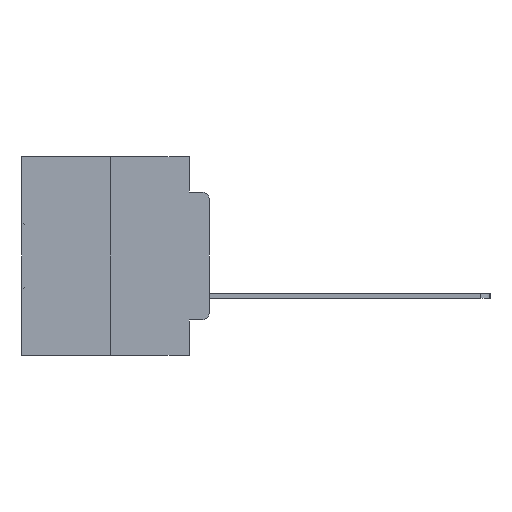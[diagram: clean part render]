
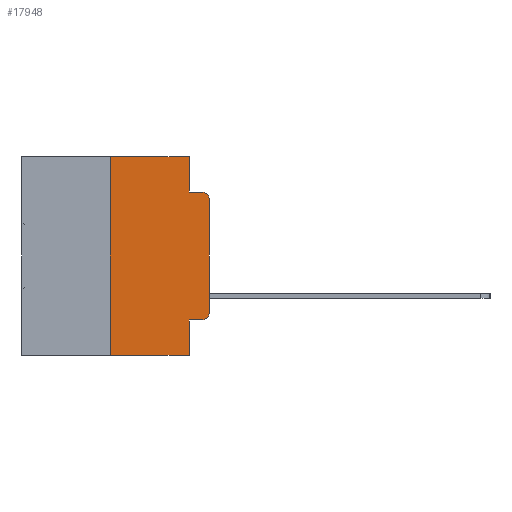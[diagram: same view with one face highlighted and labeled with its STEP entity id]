
A CAD part, left-side view. The second image highlights one B-rep face of the part: STEP entity #17948.
In plain terms, the highlighted planar face has unit normal (-1, 0, 0).
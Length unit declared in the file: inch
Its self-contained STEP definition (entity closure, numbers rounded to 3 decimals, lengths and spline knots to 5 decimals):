
#135 = CARTESIAN_POINT ( 'NONE',  ( 0., 0.473, 0. ) ) ;
#407 = EDGE_CURVE ( 'NONE', #14421, #8506, #14836, .T. ) ;
#2081 = ORIENTED_EDGE ( 'NONE', *, *, #20221, .T. ) ;
#2474 = ORIENTED_EDGE ( 'NONE', *, *, #28296, .F. ) ;
#2685 = DIRECTION ( 'NONE',  ( 0., 0., -1. ) ) ;
#2737 = EDGE_CURVE ( 'NONE', #5109, #17526, #16474, .T. ) ;
#2983 = CARTESIAN_POINT ( 'NONE',  ( 0., 0.473, 0. ) ) ;
#3558 = CARTESIAN_POINT ( 'NONE',  ( 0., 0.25, 0. ) ) ;
#3638 = ORIENTED_EDGE ( 'NONE', *, *, #28166, .T. ) ;
#5041 = EDGE_LOOP ( 'NONE', ( #15099, #5907, #12115, #9415, #2474, #17020, #29614, #31041, #2081, #3638 ) ) ;
#5109 = VERTEX_POINT ( 'NONE', #23077 ) ;
#5199 = DIRECTION ( 'NONE',  ( 0., -1., 0. ) ) ;
#5673 = DIRECTION ( 'NONE',  ( 0., 0., -1. ) ) ;
#5705 = LINE ( 'NONE', #2983, #29736 ) ;
#5858 = CARTESIAN_POINT ( 'NONE',  ( 0., 0.051, 0. ) ) ;
#5907 = ORIENTED_EDGE ( 'NONE', *, *, #24404, .T. ) ;
#5929 = LINE ( 'NONE', #17070, #24414 ) ;
#6015 = EDGE_CURVE ( 'NONE', #12512, #10675, #6375, .T. ) ;
#6375 = LINE ( 'NONE', #15417, #29650 ) ;
#6469 = AXIS2_PLACEMENT_3D ( 'NONE', #23797, #9454, #26210 ) ;
#6505 = VECTOR ( 'NONE', #11482, 39.37008 ) ;
#7074 = EDGE_CURVE ( 'NONE', #14337, #14650, #25894, .T. ) ;
#7300 = LINE ( 'NONE', #18593, #6505 ) ;
#7598 = CARTESIAN_POINT ( 'NONE',  ( 0., 0.02, -0.0885 ) ) ;
#8362 = EDGE_CURVE ( 'NONE', #5109, #8506, #5929, .T. ) ;
#8506 = VERTEX_POINT ( 'NONE', #21443 ) ;
#8847 = AXIS2_PLACEMENT_3D ( 'NONE', #24236, #9907, #26644 ) ;
#9415 = ORIENTED_EDGE ( 'NONE', *, *, #6015, .F. ) ;
#9454 = DIRECTION ( 'NONE',  ( -1., 0., 0. ) ) ;
#9532 = FACE_OUTER_BOUND ( 'NONE', #5041, .T. ) ;
#9623 = CARTESIAN_POINT ( 'NONE',  ( 0., 0., 0. ) ) ;
#9907 = DIRECTION ( 'NONE',  ( -1., 0., 0. ) ) ;
#10675 = VERTEX_POINT ( 'NONE', #19900 ) ;
#11482 = DIRECTION ( 'NONE',  ( 0., -1., 0. ) ) ;
#11987 = CARTESIAN_POINT ( 'NONE',  ( 0., 0.051, -0.4115 ) ) ;
#12115 = ORIENTED_EDGE ( 'NONE', *, *, #29924, .F. ) ;
#12512 = VERTEX_POINT ( 'NONE', #12777 ) ;
#12777 = CARTESIAN_POINT ( 'NONE',  ( 0., 0.051, 0. ) ) ;
#12924 = LINE ( 'NONE', #24522, #18495 ) ;
#14337 = VERTEX_POINT ( 'NONE', #25944 ) ;
#14421 = VERTEX_POINT ( 'NONE', #11987 ) ;
#14650 = VERTEX_POINT ( 'NONE', #15231 ) ;
#14836 = LINE ( 'NONE', #5858, #20377 ) ;
#14926 = PLANE ( 'NONE',  #19261 ) ;
#15099 = ORIENTED_EDGE ( 'NONE', *, *, #7074, .T. ) ;
#15231 = CARTESIAN_POINT ( 'NONE',  ( 0., 0., -0.1085 ) ) ;
#15417 = CARTESIAN_POINT ( 'NONE',  ( 0., 0.051, 0. ) ) ;
#15715 = VECTOR ( 'NONE', #20836, 39.37008 ) ;
#16474 = LINE ( 'NONE', #27923, #15715 ) ;
#17020 = ORIENTED_EDGE ( 'NONE', *, *, #2737, .F. ) ;
#17070 = CARTESIAN_POINT ( 'NONE',  ( 0., 0.473, -0.5 ) ) ;
#17305 = DIRECTION ( 'NONE',  ( 1., 0., 0. ) ) ;
#17526 = VERTEX_POINT ( 'NONE', #3558 ) ;
#17599 = DIRECTION ( 'NONE',  ( 0., -1., 0. ) ) ;
#17948 = ADVANCED_FACE ( 'NONE', ( #9532 ), #14926, .F. ) ;
#18495 = VECTOR ( 'NONE', #5199, 39.37008 ) ;
#18593 = CARTESIAN_POINT ( 'NONE',  ( 0., 0.051, -0.4115 ) ) ;
#19261 = AXIS2_PLACEMENT_3D ( 'NONE', #135, #17305, #2685 ) ;
#19293 = DIRECTION ( 'NONE',  ( 0., 0., 1. ) ) ;
#19563 = VECTOR ( 'NONE', #19293, 39.37008 ) ;
#19900 = CARTESIAN_POINT ( 'NONE',  ( 0., 0.051, -0.0885 ) ) ;
#19940 = VERTEX_POINT ( 'NONE', #22341 ) ;
#20117 = CIRCLE ( 'NONE', #8847, 0.02 ) ;
#20221 = EDGE_CURVE ( 'NONE', #14421, #19940, #7300, .T. ) ;
#20377 = VECTOR ( 'NONE', #30638, 39.37008 ) ;
#20836 = DIRECTION ( 'NONE',  ( 0., 0., 1. ) ) ;
#21443 = CARTESIAN_POINT ( 'NONE',  ( 0., 0.051, -0.5 ) ) ;
#22341 = CARTESIAN_POINT ( 'NONE',  ( 0., 0.02, -0.4115 ) ) ;
#23077 = CARTESIAN_POINT ( 'NONE',  ( 0., 0.25, -0.5 ) ) ;
#23255 = VERTEX_POINT ( 'NONE', #7598 ) ;
#23797 = CARTESIAN_POINT ( 'NONE',  ( 0., 0.02, -0.1085 ) ) ;
#24236 = CARTESIAN_POINT ( 'NONE',  ( 0., 0.02, -0.3915 ) ) ;
#24404 = EDGE_CURVE ( 'NONE', #14650, #23255, #28792, .T. ) ;
#24414 = VECTOR ( 'NONE', #26619, 39.37008 ) ;
#24522 = CARTESIAN_POINT ( 'NONE',  ( 0., 0.051, -0.0885 ) ) ;
#25894 = LINE ( 'NONE', #9623, #19563 ) ;
#25944 = CARTESIAN_POINT ( 'NONE',  ( 0., 0., -0.3915 ) ) ;
#26210 = DIRECTION ( 'NONE',  ( 0., 0., -1. ) ) ;
#26619 = DIRECTION ( 'NONE',  ( 0., -1., 0. ) ) ;
#26644 = DIRECTION ( 'NONE',  ( 0., 0., -1. ) ) ;
#27923 = CARTESIAN_POINT ( 'NONE',  ( 0., 0.25, 0. ) ) ;
#28166 = EDGE_CURVE ( 'NONE', #19940, #14337, #20117, .T. ) ;
#28296 = EDGE_CURVE ( 'NONE', #17526, #12512, #5705, .T. ) ;
#28792 = CIRCLE ( 'NONE', #6469, 0.02 ) ;
#29614 = ORIENTED_EDGE ( 'NONE', *, *, #8362, .T. ) ;
#29650 = VECTOR ( 'NONE', #5673, 39.37008 ) ;
#29736 = VECTOR ( 'NONE', #17599, 39.37008 ) ;
#29924 = EDGE_CURVE ( 'NONE', #10675, #23255, #12924, .T. ) ;
#30638 = DIRECTION ( 'NONE',  ( 0., 0., -1. ) ) ;
#31041 = ORIENTED_EDGE ( 'NONE', *, *, #407, .F. ) ;
